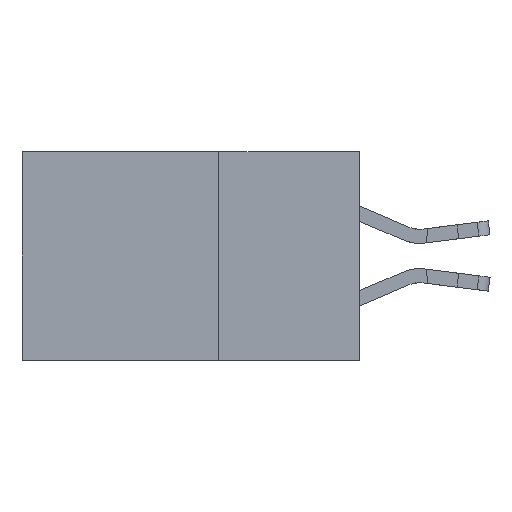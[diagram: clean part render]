
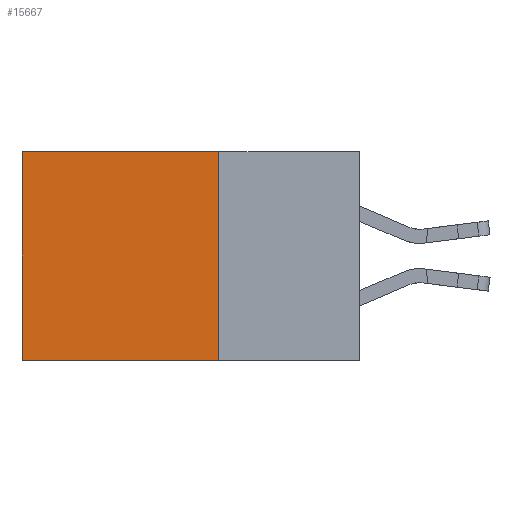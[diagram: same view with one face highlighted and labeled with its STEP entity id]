
A CAD part, left-side view. The second image highlights one B-rep face of the part: STEP entity #15667.
In plain terms, the highlighted planar face has unit normal (-1, 0, 0).
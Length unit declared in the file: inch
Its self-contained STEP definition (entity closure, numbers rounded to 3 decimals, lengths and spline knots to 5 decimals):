
#338 = DIRECTION ( 'NONE',  ( 0., 1., 0. ) ) ;
#1282 = LINE ( 'NONE', #22683, #14876 ) ;
#2006 = EDGE_CURVE ( 'NONE', #25249, #10099, #1282, .T. ) ;
#2135 = CARTESIAN_POINT ( 'NONE',  ( 0.2875, 0.25, 0. ) ) ;
#2592 = CARTESIAN_POINT ( 'NONE',  ( 0.2875, 0.6, 0. ) ) ;
#2957 = LINE ( 'NONE', #11209, #15628 ) ;
#3357 = VERTEX_POINT ( 'NONE', #2592 ) ;
#3781 = CARTESIAN_POINT ( 'NONE',  ( 0.2875, 0.6, -0.37 ) ) ;
#3796 = PLANE ( 'NONE',  #22672 ) ;
#6433 = CARTESIAN_POINT ( 'NONE',  ( 0.2875, 0.25, -0.37 ) ) ;
#7778 = CARTESIAN_POINT ( 'NONE',  ( 0.2875, 0.25, 0. ) ) ;
#9160 = VECTOR ( 'NONE', #20433, 39.37008 ) ;
#9611 = DIRECTION ( 'NONE',  ( 1., 0., 0. ) ) ;
#10084 = VECTOR ( 'NONE', #338, 39.37008 ) ;
#10099 = VERTEX_POINT ( 'NONE', #25103 ) ;
#10112 = FACE_OUTER_BOUND ( 'NONE', #21214, .T. ) ;
#10576 = DIRECTION ( 'NONE',  ( 0., 0., -1. ) ) ;
#11209 = CARTESIAN_POINT ( 'NONE',  ( 0.2875, 0.6, 0. ) ) ;
#11272 = ORIENTED_EDGE ( 'NONE', *, *, #14746, .T. ) ;
#11733 = DIRECTION ( 'NONE',  ( 0., 0., -1. ) ) ;
#13141 = EDGE_CURVE ( 'NONE', #3357, #21575, #2957, .T. ) ;
#13890 = ORIENTED_EDGE ( 'NONE', *, *, #15972, .F. ) ;
#14746 = EDGE_CURVE ( 'NONE', #25249, #3357, #23691, .T. ) ;
#14876 = VECTOR ( 'NONE', #10576, 39.37008 ) ;
#15184 = LINE ( 'NONE', #6433, #10084 ) ;
#15628 = VECTOR ( 'NONE', #21392, 39.37008 ) ;
#15667 = ADVANCED_FACE ( 'NONE', ( #10112 ), #3796, .F. ) ;
#15972 = EDGE_CURVE ( 'NONE', #10099, #21575, #15184, .T. ) ;
#20433 = DIRECTION ( 'NONE',  ( 0., 1., 0. ) ) ;
#21214 = EDGE_LOOP ( 'NONE', ( #25992, #13890, #22315, #11272 ) ) ;
#21392 = DIRECTION ( 'NONE',  ( 0., 0., -1. ) ) ;
#21575 = VERTEX_POINT ( 'NONE', #3781 ) ;
#22315 = ORIENTED_EDGE ( 'NONE', *, *, #2006, .F. ) ;
#22385 = CARTESIAN_POINT ( 'NONE',  ( 0.2875, 0.25, 0. ) ) ;
#22672 = AXIS2_PLACEMENT_3D ( 'NONE', #7778, #9611, #11733 ) ;
#22683 = CARTESIAN_POINT ( 'NONE',  ( 0.2875, 0.25, 0. ) ) ;
#23691 = LINE ( 'NONE', #2135, #9160 ) ;
#25103 = CARTESIAN_POINT ( 'NONE',  ( 0.2875, 0.25, -0.37 ) ) ;
#25249 = VERTEX_POINT ( 'NONE', #22385 ) ;
#25992 = ORIENTED_EDGE ( 'NONE', *, *, #13141, .T. ) ;
